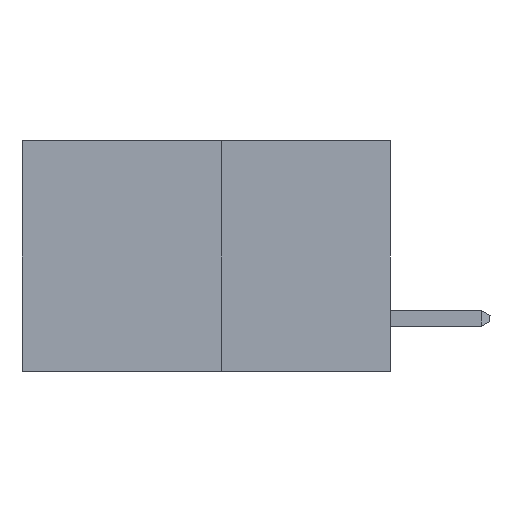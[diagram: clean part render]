
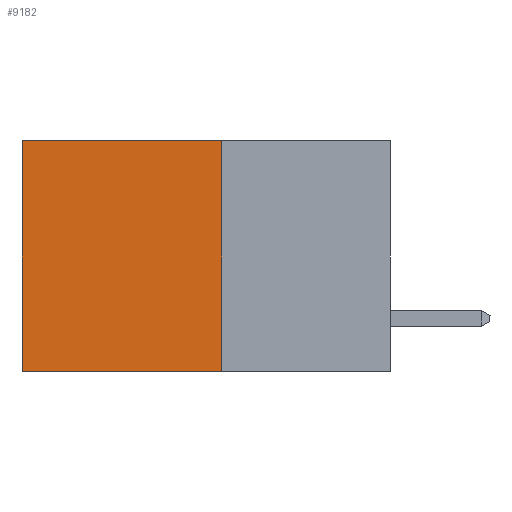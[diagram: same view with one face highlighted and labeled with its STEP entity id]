
A CAD part, left-side view. The second image highlights one B-rep face of the part: STEP entity #9182.
In plain terms, the highlighted planar face has unit normal (-1, 0, 0).
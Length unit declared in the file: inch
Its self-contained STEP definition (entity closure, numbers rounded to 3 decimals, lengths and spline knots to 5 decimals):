
#628 = DIRECTION ( 'NONE',  ( 0., 1., 0. ) ) ;
#919 = DIRECTION ( 'NONE',  ( 0., 0., -1. ) ) ;
#929 = EDGE_CURVE ( 'NONE', #6234, #8952, #1242, .T. ) ;
#1048 = ORIENTED_EDGE ( 'NONE', *, *, #929, .T. ) ;
#1106 = FACE_OUTER_BOUND ( 'NONE', #2549, .T. ) ;
#1136 = EDGE_CURVE ( 'NONE', #3940, #8952, #3591, .T. ) ;
#1242 = LINE ( 'NONE', #2800, #5858 ) ;
#1351 = ORIENTED_EDGE ( 'NONE', *, *, #11401, .T. ) ;
#1400 = VECTOR ( 'NONE', #10170, 39.37008 ) ;
#1506 = CARTESIAN_POINT ( 'NONE',  ( 0.277, 0.27, 0. ) ) ;
#1569 = DIRECTION ( 'NONE',  ( 0., 0., -1. ) ) ;
#2316 = LINE ( 'NONE', #4370, #11320 ) ;
#2549 = EDGE_LOOP ( 'NONE', ( #1048, #8271, #10491, #1351 ) ) ;
#2800 = CARTESIAN_POINT ( 'NONE',  ( 0.277, 0.59, -0.37 ) ) ;
#3591 = LINE ( 'NONE', #5489, #1400 ) ;
#3940 = VERTEX_POINT ( 'NONE', #7467 ) ;
#4087 = AXIS2_PLACEMENT_3D ( 'NONE', #11432, #6428, #919 ) ;
#4370 = CARTESIAN_POINT ( 'NONE',  ( 0.277, 0.27, 0. ) ) ;
#4650 = PLANE ( 'NONE',  #4087 ) ;
#5489 = CARTESIAN_POINT ( 'NONE',  ( 0.277, 0.27, -0.37 ) ) ;
#5858 = VECTOR ( 'NONE', #1569, 39.37008 ) ;
#5906 = EDGE_CURVE ( 'NONE', #9671, #3940, #7845, .T. ) ;
#6234 = VERTEX_POINT ( 'NONE', #7175 ) ;
#6428 = DIRECTION ( 'NONE',  ( 1., 0., 0. ) ) ;
#7175 = CARTESIAN_POINT ( 'NONE',  ( 0.277, 0.59, 0. ) ) ;
#7467 = CARTESIAN_POINT ( 'NONE',  ( 0.277, 0.27, -0.37 ) ) ;
#7572 = VECTOR ( 'NONE', #7840, 39.37008 ) ;
#7840 = DIRECTION ( 'NONE',  ( 0., 0., -1. ) ) ;
#7845 = LINE ( 'NONE', #9163, #7572 ) ;
#7901 = CARTESIAN_POINT ( 'NONE',  ( 0.277, 0.59, -0.37 ) ) ;
#8271 = ORIENTED_EDGE ( 'NONE', *, *, #1136, .F. ) ;
#8952 = VERTEX_POINT ( 'NONE', #7901 ) ;
#9163 = CARTESIAN_POINT ( 'NONE',  ( 0.277, 0.27, -0.37 ) ) ;
#9182 = ADVANCED_FACE ( 'NONE', ( #1106 ), #4650, .F. ) ;
#9671 = VERTEX_POINT ( 'NONE', #1506 ) ;
#10170 = DIRECTION ( 'NONE',  ( 0., 1., 0. ) ) ;
#10491 = ORIENTED_EDGE ( 'NONE', *, *, #5906, .F. ) ;
#11320 = VECTOR ( 'NONE', #628, 39.37008 ) ;
#11401 = EDGE_CURVE ( 'NONE', #9671, #6234, #2316, .T. ) ;
#11432 = CARTESIAN_POINT ( 'NONE',  ( 0.277, 0.27, -0.37 ) ) ;
